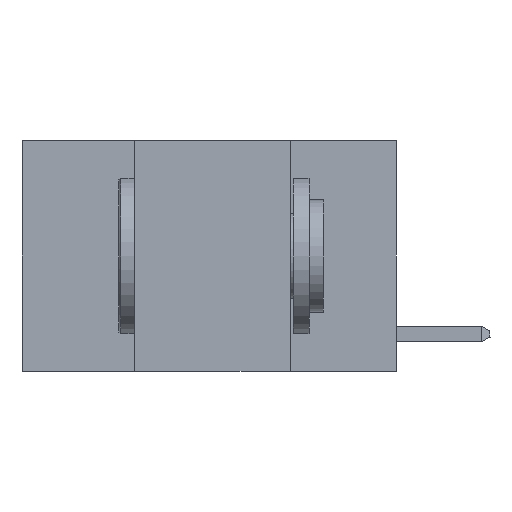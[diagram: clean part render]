
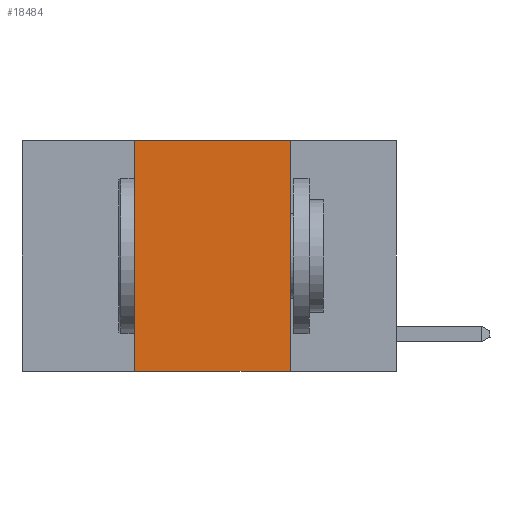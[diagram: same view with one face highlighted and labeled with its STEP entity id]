
A CAD part, left-side view. The second image highlights one B-rep face of the part: STEP entity #18484.
In plain terms, the highlighted planar face has unit normal (-1, 0, 0).
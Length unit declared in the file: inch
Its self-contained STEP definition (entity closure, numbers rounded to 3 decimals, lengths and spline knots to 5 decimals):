
#115 = ORIENTED_EDGE ( 'NONE', *, *, #25059, .F. ) ;
#299 = VECTOR ( 'NONE', #6704, 39.37008 ) ;
#315 = ORIENTED_EDGE ( 'NONE', *, *, #24545, .F. ) ;
#2070 = CARTESIAN_POINT ( 'NONE',  ( 0., 0.42, 0. ) ) ;
#3285 = AXIS2_PLACEMENT_3D ( 'NONE', #6564, #26629, #13330 ) ;
#3703 = ORIENTED_EDGE ( 'NONE', *, *, #16154, .F. ) ;
#4459 = CARTESIAN_POINT ( 'NONE',  ( 0., 0.42, 0. ) ) ;
#5014 = ORIENTED_EDGE ( 'NONE', *, *, #10116, .T. ) ;
#6564 = CARTESIAN_POINT ( 'NONE',  ( 0., 0.6, 0. ) ) ;
#6704 = DIRECTION ( 'NONE',  ( 0., 0., 1. ) ) ;
#7893 = DIRECTION ( 'NONE',  ( 0., -1., 0. ) ) ;
#8515 = VECTOR ( 'NONE', #15495, 39.37008 ) ;
#8781 = VERTEX_POINT ( 'NONE', #2070 ) ;
#8822 = PLANE ( 'NONE',  #3285 ) ;
#9621 = FACE_OUTER_BOUND ( 'NONE', #22892, .T. ) ;
#9921 = LINE ( 'NONE', #24319, #8515 ) ;
#10116 = EDGE_CURVE ( 'NONE', #23441, #14290, #17892, .T. ) ;
#12173 = CARTESIAN_POINT ( 'NONE',  ( 0., 0.17, 0. ) ) ;
#12762 = CARTESIAN_POINT ( 'NONE',  ( 0., 0.17, -0.37 ) ) ;
#13330 = DIRECTION ( 'NONE',  ( 0., 0., -1. ) ) ;
#14245 = VERTEX_POINT ( 'NONE', #12173 ) ;
#14290 = VERTEX_POINT ( 'NONE', #12762 ) ;
#15381 = CARTESIAN_POINT ( 'NONE',  ( 0., 0.17, 0. ) ) ;
#15495 = DIRECTION ( 'NONE',  ( 0., -1., 0. ) ) ;
#16154 = EDGE_CURVE ( 'NONE', #23441, #8781, #18148, .T. ) ;
#17892 = LINE ( 'NONE', #21270, #22387 ) ;
#18148 = LINE ( 'NONE', #4459, #299 ) ;
#18297 = VECTOR ( 'NONE', #19847, 39.37008 ) ;
#18484 = ADVANCED_FACE ( 'NONE', ( #9621 ), #8822, .F. ) ;
#18995 = LINE ( 'NONE', #15381, #18297 ) ;
#19847 = DIRECTION ( 'NONE',  ( 0., 0., -1. ) ) ;
#21270 = CARTESIAN_POINT ( 'NONE',  ( 0., 0.6, -0.37 ) ) ;
#22387 = VECTOR ( 'NONE', #7893, 39.37008 ) ;
#22813 = CARTESIAN_POINT ( 'NONE',  ( 0., 0.42, -0.37 ) ) ;
#22892 = EDGE_LOOP ( 'NONE', ( #115, #315, #3703, #5014 ) ) ;
#23441 = VERTEX_POINT ( 'NONE', #22813 ) ;
#24319 = CARTESIAN_POINT ( 'NONE',  ( 0., 0.6, 0. ) ) ;
#24545 = EDGE_CURVE ( 'NONE', #8781, #14245, #9921, .T. ) ;
#25059 = EDGE_CURVE ( 'NONE', #14245, #14290, #18995, .T. ) ;
#26629 = DIRECTION ( 'NONE',  ( 1., 0., 0. ) ) ;
